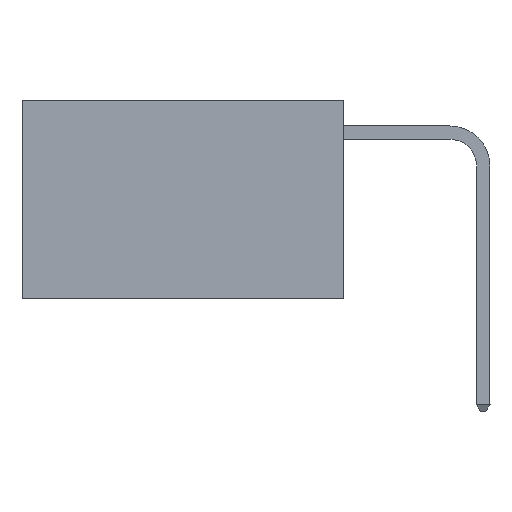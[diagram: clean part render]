
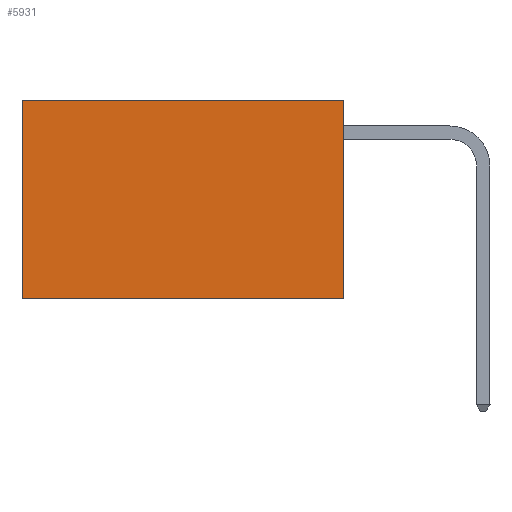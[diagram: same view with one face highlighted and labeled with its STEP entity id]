
A CAD part, left-side view. The second image highlights one B-rep face of the part: STEP entity #5931.
In plain terms, the highlighted planar face has unit normal (-1, 0, 0).
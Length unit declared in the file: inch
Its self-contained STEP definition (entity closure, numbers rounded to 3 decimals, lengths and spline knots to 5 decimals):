
#639 = VERTEX_POINT ( 'NONE', #9192 ) ;
#1420 = ORIENTED_EDGE ( 'NONE', *, *, #6879, .T. ) ;
#1553 = LINE ( 'NONE', #11053, #3840 ) ;
#2213 = FACE_OUTER_BOUND ( 'NONE', #9329, .T. ) ;
#2623 = VERTEX_POINT ( 'NONE', #8375 ) ;
#2699 = DIRECTION ( 'NONE',  ( 0., 0., -1. ) ) ;
#2901 = CARTESIAN_POINT ( 'NONE',  ( 0.2625, 0., 0. ) ) ;
#2935 = VECTOR ( 'NONE', #10095, 39.37008 ) ;
#3840 = VECTOR ( 'NONE', #6361, 39.37008 ) ;
#4053 = ORIENTED_EDGE ( 'NONE', *, *, #7898, .F. ) ;
#4371 = ORIENTED_EDGE ( 'NONE', *, *, #4424, .F. ) ;
#4424 = EDGE_CURVE ( 'NONE', #5026, #639, #7746, .T. ) ;
#5026 = VERTEX_POINT ( 'NONE', #2901 ) ;
#5377 = ORIENTED_EDGE ( 'NONE', *, *, #6836, .T. ) ;
#5872 = CARTESIAN_POINT ( 'NONE',  ( 0.2625, 0.6, 0. ) ) ;
#5931 = ADVANCED_FACE ( 'NONE', ( #2213 ), #12396, .F. ) ;
#6361 = DIRECTION ( 'NONE',  ( 0., 1., 0. ) ) ;
#6572 = VECTOR ( 'NONE', #8064, 39.37008 ) ;
#6836 = EDGE_CURVE ( 'NONE', #5026, #12325, #11586, .T. ) ;
#6879 = EDGE_CURVE ( 'NONE', #12325, #2623, #10700, .T. ) ;
#7106 = CARTESIAN_POINT ( 'NONE',  ( 0.2625, 0., 0. ) ) ;
#7746 = LINE ( 'NONE', #10390, #8357 ) ;
#7898 = EDGE_CURVE ( 'NONE', #639, #2623, #1553, .T. ) ;
#8064 = DIRECTION ( 'NONE',  ( 0., 1., 0. ) ) ;
#8357 = VECTOR ( 'NONE', #8523, 39.37008 ) ;
#8375 = CARTESIAN_POINT ( 'NONE',  ( 0.2625, 0.6, -0.37 ) ) ;
#8523 = DIRECTION ( 'NONE',  ( 0., 0., -1. ) ) ;
#8607 = DIRECTION ( 'NONE',  ( 1., 0., 0. ) ) ;
#9139 = CARTESIAN_POINT ( 'NONE',  ( 0.2625, 0.6, 0. ) ) ;
#9192 = CARTESIAN_POINT ( 'NONE',  ( 0.2625, 0., -0.37 ) ) ;
#9329 = EDGE_LOOP ( 'NONE', ( #1420, #4053, #4371, #5377 ) ) ;
#10095 = DIRECTION ( 'NONE',  ( 0., 0., -1. ) ) ;
#10390 = CARTESIAN_POINT ( 'NONE',  ( 0.2625, 0., 0. ) ) ;
#10392 = AXIS2_PLACEMENT_3D ( 'NONE', #10467, #8607, #2699 ) ;
#10467 = CARTESIAN_POINT ( 'NONE',  ( 0.2625, 0., 0. ) ) ;
#10700 = LINE ( 'NONE', #9139, #2935 ) ;
#11053 = CARTESIAN_POINT ( 'NONE',  ( 0.2625, 0., -0.37 ) ) ;
#11586 = LINE ( 'NONE', #7106, #6572 ) ;
#12325 = VERTEX_POINT ( 'NONE', #5872 ) ;
#12396 = PLANE ( 'NONE',  #10392 ) ;
